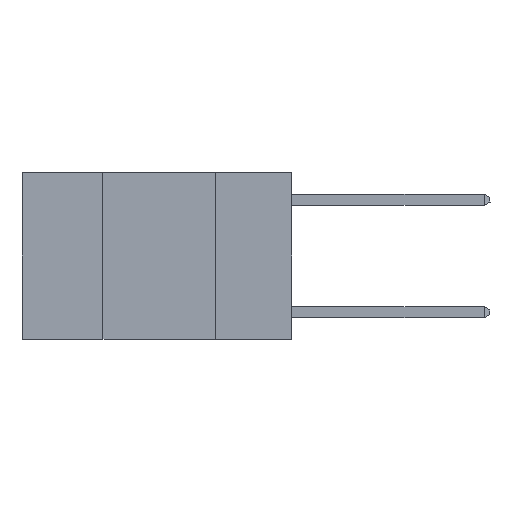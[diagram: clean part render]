
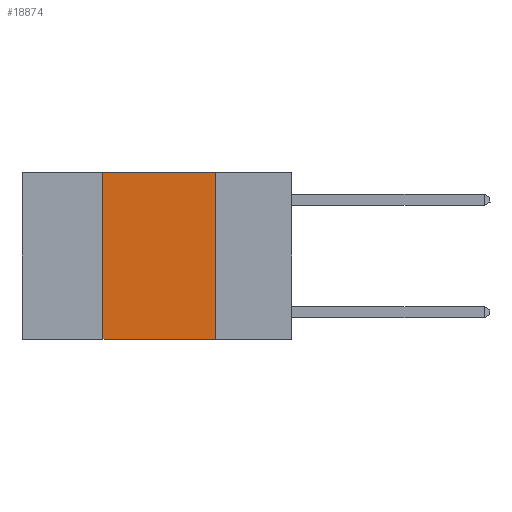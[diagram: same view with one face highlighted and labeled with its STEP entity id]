
A CAD part, left-side view. The second image highlights one B-rep face of the part: STEP entity #18874.
In plain terms, the highlighted planar face has unit normal (-1, 0, 0).
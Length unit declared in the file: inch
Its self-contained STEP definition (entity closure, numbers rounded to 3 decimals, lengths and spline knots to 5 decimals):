
#253 = CARTESIAN_POINT ( 'NONE',  ( 0., 0.6, -0.37 ) ) ;
#636 = VERTEX_POINT ( 'NONE', #6246 ) ;
#1299 = FACE_OUTER_BOUND ( 'NONE', #11976, .T. ) ;
#1571 = VERTEX_POINT ( 'NONE', #6605 ) ;
#3970 = CARTESIAN_POINT ( 'NONE',  ( 0., 0.42, -0.37 ) ) ;
#5364 = LINE ( 'NONE', #253, #15181 ) ;
#5639 = DIRECTION ( 'NONE',  ( 0., 0., -1. ) ) ;
#5876 = CARTESIAN_POINT ( 'NONE',  ( 0., 0.6, 0. ) ) ;
#6246 = CARTESIAN_POINT ( 'NONE',  ( 0., 0.17, -0.37 ) ) ;
#6277 = CARTESIAN_POINT ( 'NONE',  ( 0., 0.42, 0. ) ) ;
#6605 = CARTESIAN_POINT ( 'NONE',  ( 0., 0.17, 0. ) ) ;
#6761 = EDGE_CURVE ( 'NONE', #7229, #19476, #20710, .T. ) ;
#7229 = VERTEX_POINT ( 'NONE', #3970 ) ;
#7870 = DIRECTION ( 'NONE',  ( 0., 0., -1. ) ) ;
#8063 = VECTOR ( 'NONE', #5639, 39.37008 ) ;
#8081 = EDGE_CURVE ( 'NONE', #1571, #636, #17862, .T. ) ;
#9817 = AXIS2_PLACEMENT_3D ( 'NONE', #5876, #19654, #7870 ) ;
#11521 = ORIENTED_EDGE ( 'NONE', *, *, #8081, .F. ) ;
#11976 = EDGE_LOOP ( 'NONE', ( #11521, #13009, #25249, #13896 ) ) ;
#13009 = ORIENTED_EDGE ( 'NONE', *, *, #18795, .F. ) ;
#13518 = CARTESIAN_POINT ( 'NONE',  ( 0., 0.17, 0. ) ) ;
#13662 = LINE ( 'NONE', #17472, #18312 ) ;
#13896 = ORIENTED_EDGE ( 'NONE', *, *, #25152, .T. ) ;
#15181 = VECTOR ( 'NONE', #16131, 39.37008 ) ;
#15353 = CARTESIAN_POINT ( 'NONE',  ( 0., 0.42, 0. ) ) ;
#15470 = DIRECTION ( 'NONE',  ( 0., -1., 0. ) ) ;
#16131 = DIRECTION ( 'NONE',  ( 0., -1., 0. ) ) ;
#16698 = VECTOR ( 'NONE', #23980, 39.37008 ) ;
#17472 = CARTESIAN_POINT ( 'NONE',  ( 0., 0.6, 0. ) ) ;
#17862 = LINE ( 'NONE', #13518, #8063 ) ;
#18312 = VECTOR ( 'NONE', #15470, 39.37008 ) ;
#18795 = EDGE_CURVE ( 'NONE', #19476, #1571, #13662, .T. ) ;
#18874 = ADVANCED_FACE ( 'NONE', ( #1299 ), #23507, .F. ) ;
#19476 = VERTEX_POINT ( 'NONE', #15353 ) ;
#19654 = DIRECTION ( 'NONE',  ( 1., 0., 0. ) ) ;
#20710 = LINE ( 'NONE', #6277, #16698 ) ;
#23507 = PLANE ( 'NONE',  #9817 ) ;
#23980 = DIRECTION ( 'NONE',  ( 0., 0., 1. ) ) ;
#25152 = EDGE_CURVE ( 'NONE', #7229, #636, #5364, .T. ) ;
#25249 = ORIENTED_EDGE ( 'NONE', *, *, #6761, .F. ) ;
